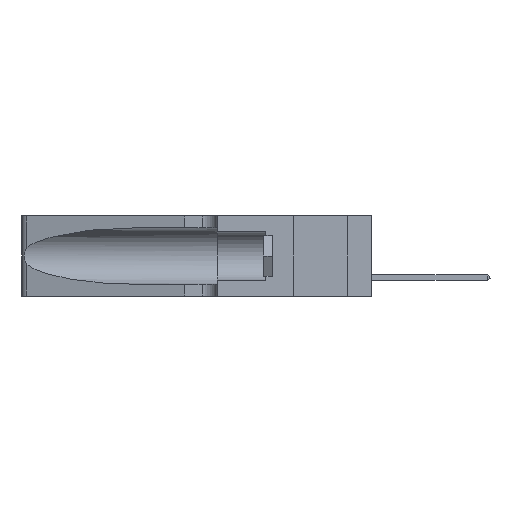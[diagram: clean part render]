
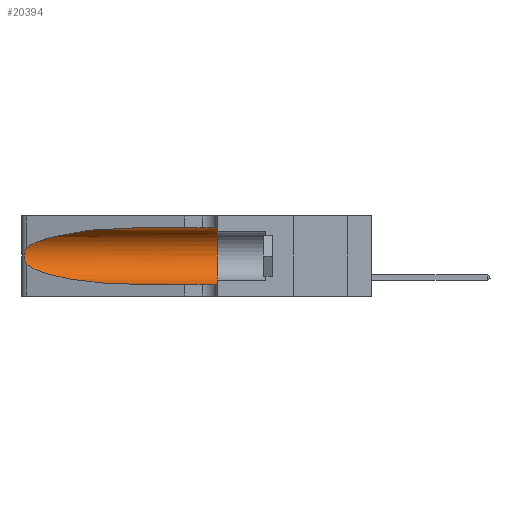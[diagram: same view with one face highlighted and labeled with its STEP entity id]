
A CAD part, left-side view. The second image highlights one B-rep face of the part: STEP entity #20394.
In plain terms, the highlighted cylindrical face has radius 3.308 mm (diameter 6.617 mm), a partial arc.
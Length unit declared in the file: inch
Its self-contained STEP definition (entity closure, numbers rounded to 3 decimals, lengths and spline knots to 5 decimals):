
#945 = CARTESIAN_POINT ( 'NONE',  ( 0.25856, 1.23593, 0.16098 ) ) ;
#1303 = AXIS2_PLACEMENT_3D ( 'NONE', #25011, #24873, #27634 ) ;
#1456 = EDGE_CURVE ( 'NONE', #28396, #4563, #23261, .T. ) ;
#1821 = CARTESIAN_POINT ( 'NONE',  ( 0.1305, 0.35, 0.31525 ) ) ;
#2549 = EDGE_CURVE ( 'NONE', #20098, #9798, #3953, .T. ) ;
#3451 = CARTESIAN_POINT ( 'NONE',  ( 0.25487, 1.22718, 0.14631 ) ) ;
#3513 = CARTESIAN_POINT ( 'NONE',  ( 0.25639, 1.23186, 0.15144 ) ) ;
#3953 =( BOUNDED_CURVE ( )  B_SPLINE_CURVE ( 3, ( #3451, #29962, #32402, #17677 ),
 .UNSPECIFIED., .F., .T. ) 
 B_SPLINE_CURVE_WITH_KNOTS ( ( 4, 4 ),
 ( 3.44316, 4.71239 ),
 .UNSPECIFIED. ) 
 CURVE ( )  GEOMETRIC_REPRESENTATION_ITEM ( )  RATIONAL_B_SPLINE_CURVE ( ( 1., 0.87, 0.87, 1. ) ) 
 REPRESENTATION_ITEM ( '' )  );
#4563 = VERTEX_POINT ( 'NONE', #1821 ) ;
#4813 = VECTOR ( 'NONE', #11999, 39.37008 ) ;
#5201 = CIRCLE ( 'NONE', #19455, 0.13025 ) ;
#5304 = CARTESIAN_POINT ( 'NONE',  ( 0.26018, 1.23835, 0.19895 ) ) ;
#6224 = CARTESIAN_POINT ( 'NONE',  ( 0.25555, 1.22993, 0.14849 ) ) ;
#8249 = CARTESIAN_POINT ( 'NONE',  ( 0.26075, 1.23896, 0.19203 ) ) ;
#8452 =( BOUNDED_CURVE ( )  B_SPLINE_CURVE ( 3, ( #21271, #10740, #16048, #18611 ),
 .UNSPECIFIED., .F., .F. ) 
 B_SPLINE_CURVE_WITH_KNOTS ( ( 4, 4 ),
 ( 1.5708, 2.84003 ),
 .UNSPECIFIED. ) 
 CURVE ( )  GEOMETRIC_REPRESENTATION_ITEM ( )  RATIONAL_B_SPLINE_CURVE ( ( 1., 0.87, 0.87, 1. ) ) 
 REPRESENTATION_ITEM ( '' )  );
#9153 = CARTESIAN_POINT ( 'NONE',  ( 0.25487, 1.22718, 0.14631 ) ) ;
#9451 = CARTESIAN_POINT ( 'NONE',  ( 0.1305, 0.72297, 0.31525 ) ) ;
#9798 = VERTEX_POINT ( 'NONE', #23697 ) ;
#9961 = CARTESIAN_POINT ( 'NONE',  ( 0.25487, 1.22718, 0.22369 ) ) ;
#10740 = CARTESIAN_POINT ( 'NONE',  ( 0.18966, 0.96281, 0.31525 ) ) ;
#11356 = CARTESIAN_POINT ( 'NONE',  ( 0.25787, 1.23484, 0.2124 ) ) ;
#11999 = DIRECTION ( 'NONE',  ( 0., -1., 0. ) ) ;
#12146 = EDGE_CURVE ( 'NONE', #9798, #25701, #13431, .T. ) ;
#13047 = VECTOR ( 'NONE', #15188, 39.37008 ) ;
#13173 = CARTESIAN_POINT ( 'NONE',  ( 0.1305, 0.35, 0.05475 ) ) ;
#13253 = CARTESIAN_POINT ( 'NONE',  ( 0.1305, 0.35, 0.185 ) ) ;
#13431 = LINE ( 'NONE', #25411, #13047 ) ;
#15188 = DIRECTION ( 'NONE',  ( 0., -1., 0. ) ) ;
#15502 = B_SPLINE_CURVE_WITH_KNOTS ( 'NONE', 3,
 ( #9961, #23830, #20984, #11356, #32720, #5304, #8249, #21256, #16265, #945, #24099, #3513, #6224, #9153 ),
 .UNSPECIFIED., .F., .F.,
 ( 4, 2, 2, 2, 2, 2, 4 ),
 ( 0., 0.00027, 0.00053, 0.00107, 0.0016, 0.00187, 0.00214 ),
 .UNSPECIFIED. ) ;
#16048 = CARTESIAN_POINT ( 'NONE',  ( 0.2373, 1.15595, 0.28018 ) ) ;
#16265 = CARTESIAN_POINT ( 'NONE',  ( 0.26017, 1.23833, 0.17102 ) ) ;
#16710 = ORIENTED_EDGE ( 'NONE', *, *, #12146, .T. ) ;
#16831 = CYLINDRICAL_SURFACE ( 'NONE', #1303, 0.13025 ) ;
#17677 = CARTESIAN_POINT ( 'NONE',  ( 0.1305, 0.72297, 0.05475 ) ) ;
#18115 = EDGE_LOOP ( 'NONE', ( #29403, #20368, #30562, #16710, #26682, #19483 ) ) ;
#18611 = CARTESIAN_POINT ( 'NONE',  ( 0.25487, 1.22718, 0.22369 ) ) ;
#19137 = EDGE_CURVE ( 'NONE', #30905, #20098, #15502, .T. ) ;
#19455 = AXIS2_PLACEMENT_3D ( 'NONE', #13253, #20651, #20981 ) ;
#19483 = ORIENTED_EDGE ( 'NONE', *, *, #1456, .F. ) ;
#20098 = VERTEX_POINT ( 'NONE', #25821 ) ;
#20368 = ORIENTED_EDGE ( 'NONE', *, *, #19137, .T. ) ;
#20394 = ADVANCED_FACE ( 'NONE', ( #24917 ), #16831, .F. ) ;
#20651 = DIRECTION ( 'NONE',  ( 0., 1., 0. ) ) ;
#20981 = DIRECTION ( 'NONE',  ( 0., 0., 1. ) ) ;
#20984 = CARTESIAN_POINT ( 'NONE',  ( 0.25639, 1.23184, 0.21858 ) ) ;
#21256 = CARTESIAN_POINT ( 'NONE',  ( 0.26075, 1.23896, 0.178 ) ) ;
#21271 = CARTESIAN_POINT ( 'NONE',  ( 0.1305, 0.72297, 0.31525 ) ) ;
#23261 = LINE ( 'NONE', #32353, #4813 ) ;
#23697 = CARTESIAN_POINT ( 'NONE',  ( 0.1305, 0.72297, 0.05475 ) ) ;
#23830 = CARTESIAN_POINT ( 'NONE',  ( 0.25555, 1.22994, 0.2215 ) ) ;
#24099 = CARTESIAN_POINT ( 'NONE',  ( 0.25789, 1.23486, 0.15765 ) ) ;
#24415 = EDGE_CURVE ( 'NONE', #28396, #30905, #8452, .T. ) ;
#24873 = DIRECTION ( 'NONE',  ( 0., -1., 0. ) ) ;
#24917 = FACE_OUTER_BOUND ( 'NONE', #18115, .T. ) ;
#25011 = CARTESIAN_POINT ( 'NONE',  ( 0.1305, 1.61858, 0.185 ) ) ;
#25411 = CARTESIAN_POINT ( 'NONE',  ( 0.1305, 1.61858, 0.05475 ) ) ;
#25701 = VERTEX_POINT ( 'NONE', #13173 ) ;
#25821 = CARTESIAN_POINT ( 'NONE',  ( 0.25487, 1.22718, 0.14631 ) ) ;
#26682 = ORIENTED_EDGE ( 'NONE', *, *, #28118, .F. ) ;
#27634 = DIRECTION ( 'NONE',  ( 0., 0., -1. ) ) ;
#28118 = EDGE_CURVE ( 'NONE', #4563, #25701, #5201, .T. ) ;
#28396 = VERTEX_POINT ( 'NONE', #9451 ) ;
#29403 = ORIENTED_EDGE ( 'NONE', *, *, #24415, .T. ) ;
#29962 = CARTESIAN_POINT ( 'NONE',  ( 0.2373, 1.15595, 0.08982 ) ) ;
#30041 = CARTESIAN_POINT ( 'NONE',  ( 0.25487, 1.22718, 0.22369 ) ) ;
#30562 = ORIENTED_EDGE ( 'NONE', *, *, #2549, .T. ) ;
#30905 = VERTEX_POINT ( 'NONE', #30041 ) ;
#32353 = CARTESIAN_POINT ( 'NONE',  ( 0.1305, 1.61858, 0.31525 ) ) ;
#32402 = CARTESIAN_POINT ( 'NONE',  ( 0.18966, 0.96281, 0.05475 ) ) ;
#32720 = CARTESIAN_POINT ( 'NONE',  ( 0.25854, 1.2359, 0.20912 ) ) ;
